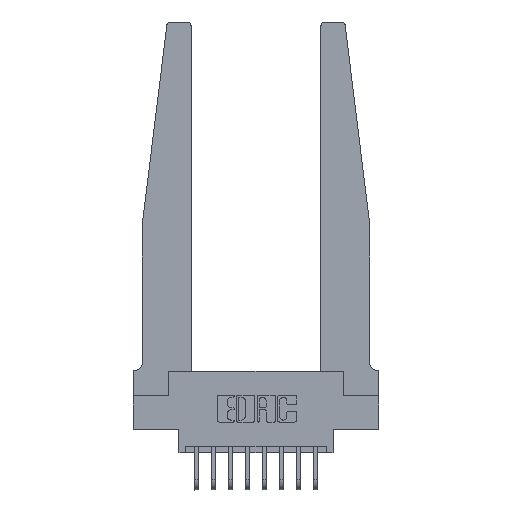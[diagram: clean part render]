
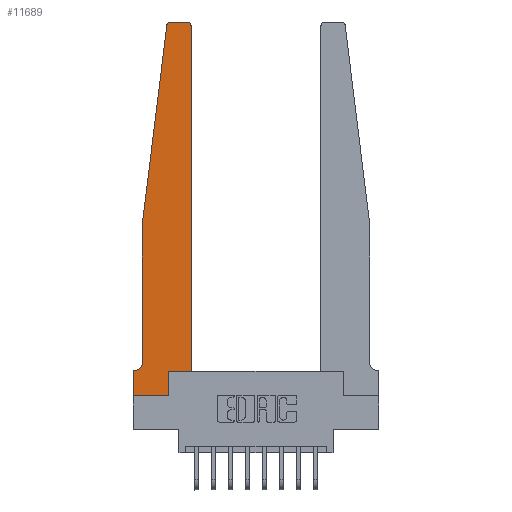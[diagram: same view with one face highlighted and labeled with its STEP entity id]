
A CAD part, top view. The second image highlights one B-rep face of the part: STEP entity #11689.
In plain terms, the highlighted planar face has unit normal (0, 0, 1).
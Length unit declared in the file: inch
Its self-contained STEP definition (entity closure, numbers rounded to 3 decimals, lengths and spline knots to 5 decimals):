
#113 = ORIENTED_EDGE ( 'NONE', *, *, #3034, .T. ) ;
#203 = CARTESIAN_POINT ( 'NONE',  ( 0.065, 1.25, 0.37 ) ) ;
#670 = LINE ( 'NONE', #2782, #13077 ) ;
#933 = CARTESIAN_POINT ( 'NONE',  ( 0.065, 0.1875, 0.37 ) ) ;
#1384 = CARTESIAN_POINT ( 'NONE',  ( 0., 0., 0.37 ) ) ;
#1413 = CARTESIAN_POINT ( 'NONE',  ( 0.2605, 0.18, 0.37 ) ) ;
#1460 = DIRECTION ( 'NONE',  ( 1., 0., 0. ) ) ;
#1673 = LINE ( 'NONE', #10899, #11116 ) ;
#1698 = CARTESIAN_POINT ( 'NONE',  ( 0.065, 1.25, 0.37 ) ) ;
#1770 = EDGE_CURVE ( 'NONE', #2819, #8285, #10843, .T. ) ;
#1806 = CARTESIAN_POINT ( 'NONE',  ( 0.425, 0.18, 0.37 ) ) ;
#1832 = CARTESIAN_POINT ( 'NONE',  ( 0.065, 1.25, 0.37 ) ) ;
#1840 = CARTESIAN_POINT ( 'NONE',  ( 0., 0.1875, 0.37 ) ) ;
#1846 = CARTESIAN_POINT ( 'NONE',  ( 0., 0., 0.37 ) ) ;
#1923 = VERTEX_POINT ( 'NONE', #2390 ) ;
#1941 = VECTOR ( 'NONE', #7293, 39.37008 ) ;
#2170 = VECTOR ( 'NONE', #9995, 39.37008 ) ;
#2390 = CARTESIAN_POINT ( 'NONE',  ( 0.395, 2.75, 0.37 ) ) ;
#2571 = DIRECTION ( 'NONE',  ( 1., 0., 0. ) ) ;
#2591 = VERTEX_POINT ( 'NONE', #1840 ) ;
#2738 = DIRECTION ( 'NONE',  ( 1., 0., 0. ) ) ;
#2782 = CARTESIAN_POINT ( 'NONE',  ( 0., 0., 0.37 ) ) ;
#2819 = VERTEX_POINT ( 'NONE', #8457 ) ;
#3034 = EDGE_CURVE ( 'NONE', #14490, #6100, #13315, .T. ) ;
#3191 = ORIENTED_EDGE ( 'NONE', *, *, #12056, .T. ) ;
#3349 = ORIENTED_EDGE ( 'NONE', *, *, #4241, .T. ) ;
#3844 = CARTESIAN_POINT ( 'NONE',  ( 0.27653, 2.72, 0.37 ) ) ;
#3982 = EDGE_CURVE ( 'NONE', #7918, #14490, #13122, .T. ) ;
#4048 = LINE ( 'NONE', #13403, #4445 ) ;
#4241 = EDGE_CURVE ( 'NONE', #10192, #6863, #12523, .T. ) ;
#4265 = AXIS2_PLACEMENT_3D ( 'NONE', #9512, #15503, #2738 ) ;
#4445 = VECTOR ( 'NONE', #5831, 39.37008 ) ;
#4564 = AXIS2_PLACEMENT_3D ( 'NONE', #3844, #15403, #1460 ) ;
#4950 = DIRECTION ( 'NONE',  ( 0., 1., 0. ) ) ;
#5351 = EDGE_CURVE ( 'NONE', #2591, #10192, #670, .T. ) ;
#5600 = EDGE_CURVE ( 'NONE', #1923, #6292, #4048, .T. ) ;
#5652 = AXIS2_PLACEMENT_3D ( 'NONE', #13741, #11339, #2571 ) ;
#5831 = DIRECTION ( 'NONE',  ( -1., 0., 0. ) ) ;
#6100 = VERTEX_POINT ( 'NONE', #13715 ) ;
#6292 = VERTEX_POINT ( 'NONE', #8226 ) ;
#6489 = ORIENTED_EDGE ( 'NONE', *, *, #7625, .T. ) ;
#6536 = CARTESIAN_POINT ( 'NONE',  ( 0.015, 0.2375, 0.37 ) ) ;
#6568 = ORIENTED_EDGE ( 'NONE', *, *, #7941, .T. ) ;
#6710 = CIRCLE ( 'NONE', #4564, 0.03 ) ;
#6863 = VERTEX_POINT ( 'NONE', #15079 ) ;
#7293 = DIRECTION ( 'NONE',  ( -0.122, -0.992, 0. ) ) ;
#7392 = FACE_OUTER_BOUND ( 'NONE', #12750, .T. ) ;
#7473 = VECTOR ( 'NONE', #13224, 39.37008 ) ;
#7625 = EDGE_CURVE ( 'NONE', #7993, #1923, #8197, .T. ) ;
#7669 = ORIENTED_EDGE ( 'NONE', *, *, #13849, .T. ) ;
#7918 = VERTEX_POINT ( 'NONE', #12310 ) ;
#7941 = EDGE_CURVE ( 'NONE', #6863, #2819, #8633, .T. ) ;
#7993 = VERTEX_POINT ( 'NONE', #8004 ) ;
#8004 = CARTESIAN_POINT ( 'NONE',  ( 0.425, 2.72, 0.37 ) ) ;
#8197 = CIRCLE ( 'NONE', #4265, 0.03 ) ;
#8226 = CARTESIAN_POINT ( 'NONE',  ( 0.27653, 2.75, 0.37 ) ) ;
#8285 = VERTEX_POINT ( 'NONE', #8511 ) ;
#8409 = CIRCLE ( 'NONE', #11135, 0.05 ) ;
#8457 = CARTESIAN_POINT ( 'NONE',  ( 0.2605, 0.18, 0.37 ) ) ;
#8511 = CARTESIAN_POINT ( 'NONE',  ( 0.425, 0.18, 0.37 ) ) ;
#8633 = LINE ( 'NONE', #1413, #15034 ) ;
#8777 = PLANE ( 'NONE',  #5652 ) ;
#8978 = LINE ( 'NONE', #933, #2170 ) ;
#9040 = DIRECTION ( 'NONE',  ( -1., 0., 0. ) ) ;
#9143 = EDGE_CURVE ( 'NONE', #10607, #2591, #8978, .T. ) ;
#9166 = DIRECTION ( 'NONE',  ( 0., 1., 0. ) ) ;
#9424 = ORIENTED_EDGE ( 'NONE', *, *, #5351, .T. ) ;
#9512 = CARTESIAN_POINT ( 'NONE',  ( 0.395, 2.72, 0.37 ) ) ;
#9800 = CARTESIAN_POINT ( 'NONE',  ( 0.015, 0.1875, 0.37 ) ) ;
#9995 = DIRECTION ( 'NONE',  ( -1., 0., 0. ) ) ;
#10192 = VERTEX_POINT ( 'NONE', #1384 ) ;
#10607 = VERTEX_POINT ( 'NONE', #9800 ) ;
#10843 = LINE ( 'NONE', #1806, #7473 ) ;
#10899 = CARTESIAN_POINT ( 'NONE',  ( 0.425, 0.18, 0.37 ) ) ;
#11116 = VECTOR ( 'NONE', #9166, 39.37008 ) ;
#11135 = AXIS2_PLACEMENT_3D ( 'NONE', #6536, #15496, #9040 ) ;
#11157 = VECTOR ( 'NONE', #15258, 39.37008 ) ;
#11339 = DIRECTION ( 'NONE',  ( 0., 0., 1. ) ) ;
#11534 = VECTOR ( 'NONE', #14590, 39.37008 ) ;
#11689 = ADVANCED_FACE ( 'NONE', ( #7392 ), #8777, .T. ) ;
#12056 = EDGE_CURVE ( 'NONE', #8285, #7993, #1673, .T. ) ;
#12310 = CARTESIAN_POINT ( 'NONE',  ( 0.24675, 2.72367, 0.37 ) ) ;
#12523 = LINE ( 'NONE', #1846, #11534 ) ;
#12750 = EDGE_LOOP ( 'NONE', ( #15192, #13660, #13019, #113, #7669, #14521, #9424, #3349, #6568, #15293, #3191, #6489 ) ) ;
#13019 = ORIENTED_EDGE ( 'NONE', *, *, #3982, .T. ) ;
#13077 = VECTOR ( 'NONE', #14331, 39.37008 ) ;
#13122 = LINE ( 'NONE', #203, #1941 ) ;
#13224 = DIRECTION ( 'NONE',  ( 1., 0., 0. ) ) ;
#13315 = LINE ( 'NONE', #1698, #11157 ) ;
#13403 = CARTESIAN_POINT ( 'NONE',  ( 0.25, 2.75, 0.37 ) ) ;
#13660 = ORIENTED_EDGE ( 'NONE', *, *, #14390, .T. ) ;
#13715 = CARTESIAN_POINT ( 'NONE',  ( 0.065, 0.2375, 0.37 ) ) ;
#13741 = CARTESIAN_POINT ( 'NONE',  ( 0., 0.1875, 0.37 ) ) ;
#13849 = EDGE_CURVE ( 'NONE', #6100, #10607, #8409, .T. ) ;
#14331 = DIRECTION ( 'NONE',  ( 0., -1., 0. ) ) ;
#14390 = EDGE_CURVE ( 'NONE', #6292, #7918, #6710, .T. ) ;
#14490 = VERTEX_POINT ( 'NONE', #1832 ) ;
#14521 = ORIENTED_EDGE ( 'NONE', *, *, #9143, .T. ) ;
#14590 = DIRECTION ( 'NONE',  ( 1., 0., 0. ) ) ;
#15034 = VECTOR ( 'NONE', #4950, 39.37008 ) ;
#15079 = CARTESIAN_POINT ( 'NONE',  ( 0.2605, 0., 0.37 ) ) ;
#15192 = ORIENTED_EDGE ( 'NONE', *, *, #5600, .T. ) ;
#15258 = DIRECTION ( 'NONE',  ( 0., -1., 0. ) ) ;
#15293 = ORIENTED_EDGE ( 'NONE', *, *, #1770, .T. ) ;
#15403 = DIRECTION ( 'NONE',  ( 0., 0., 1. ) ) ;
#15496 = DIRECTION ( 'NONE',  ( 0., 0., -1. ) ) ;
#15503 = DIRECTION ( 'NONE',  ( 0., 0., 1. ) ) ;
